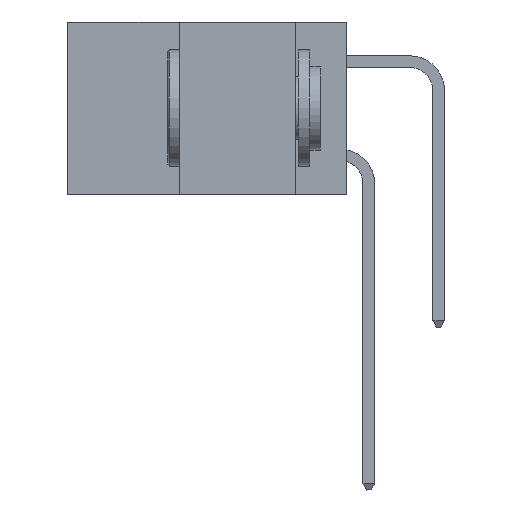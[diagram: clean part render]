
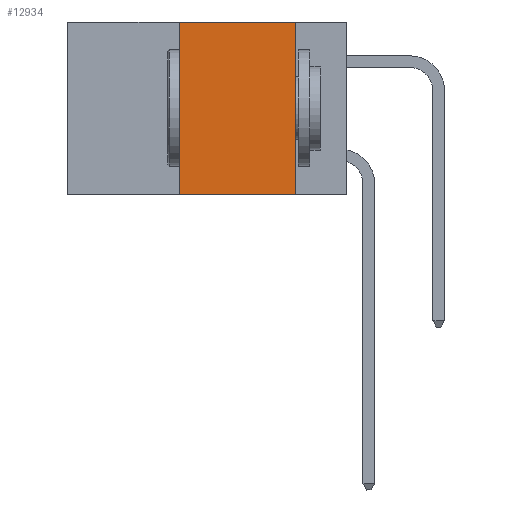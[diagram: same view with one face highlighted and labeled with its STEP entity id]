
A CAD part, left-side view. The second image highlights one B-rep face of the part: STEP entity #12934.
In plain terms, the highlighted planar face has unit normal (-1, 0, 0).
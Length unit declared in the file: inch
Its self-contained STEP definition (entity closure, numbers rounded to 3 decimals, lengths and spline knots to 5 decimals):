
#937 = LINE ( 'NONE', #5071, #10437 ) ;
#1653 = CARTESIAN_POINT ( 'NONE',  ( 0., 0.6, 0. ) ) ;
#1848 = CARTESIAN_POINT ( 'NONE',  ( 0., 0.36, 0. ) ) ;
#2266 = PLANE ( 'NONE',  #3835 ) ;
#2407 = ORIENTED_EDGE ( 'NONE', *, *, #3646, .F. ) ;
#2418 = CARTESIAN_POINT ( 'NONE',  ( 0., 0.11, 0. ) ) ;
#3545 = CARTESIAN_POINT ( 'NONE',  ( 0., 0.6, -0.37 ) ) ;
#3646 = EDGE_CURVE ( 'NONE', #12862, #16144, #12461, .T. ) ;
#3835 = AXIS2_PLACEMENT_3D ( 'NONE', #6542, #8156, #15404 ) ;
#4477 = EDGE_LOOP ( 'NONE', ( #12619, #5228, #2407, #12202 ) ) ;
#4644 = VECTOR ( 'NONE', #6473, 39.37008 ) ;
#5071 = CARTESIAN_POINT ( 'NONE',  ( 0., 0.11, 0. ) ) ;
#5228 = ORIENTED_EDGE ( 'NONE', *, *, #18281, .F. ) ;
#5990 = VECTOR ( 'NONE', #11857, 39.37008 ) ;
#6060 = VERTEX_POINT ( 'NONE', #8138 ) ;
#6473 = DIRECTION ( 'NONE',  ( 0., -1., 0. ) ) ;
#6542 = CARTESIAN_POINT ( 'NONE',  ( 0., 0.6, 0. ) ) ;
#7237 = VECTOR ( 'NONE', #7611, 39.37008 ) ;
#7611 = DIRECTION ( 'NONE',  ( 0., -1., 0. ) ) ;
#8138 = CARTESIAN_POINT ( 'NONE',  ( 0., 0.11, -0.37 ) ) ;
#8156 = DIRECTION ( 'NONE',  ( 1., 0., 0. ) ) ;
#9830 = VERTEX_POINT ( 'NONE', #2418 ) ;
#9888 = FACE_OUTER_BOUND ( 'NONE', #4477, .T. ) ;
#10437 = VECTOR ( 'NONE', #15437, 39.37008 ) ;
#11857 = DIRECTION ( 'NONE',  ( 0., 0., 1. ) ) ;
#12202 = ORIENTED_EDGE ( 'NONE', *, *, #15546, .T. ) ;
#12461 = LINE ( 'NONE', #13523, #5990 ) ;
#12619 = ORIENTED_EDGE ( 'NONE', *, *, #16235, .F. ) ;
#12862 = VERTEX_POINT ( 'NONE', #13082 ) ;
#12934 = ADVANCED_FACE ( 'NONE', ( #9888 ), #2266, .F. ) ;
#13082 = CARTESIAN_POINT ( 'NONE',  ( 0., 0.36, -0.37 ) ) ;
#13523 = CARTESIAN_POINT ( 'NONE',  ( 0., 0.36, 0. ) ) ;
#13930 = LINE ( 'NONE', #1653, #7237 ) ;
#15404 = DIRECTION ( 'NONE',  ( 0., 0., -1. ) ) ;
#15437 = DIRECTION ( 'NONE',  ( 0., 0., -1. ) ) ;
#15546 = EDGE_CURVE ( 'NONE', #12862, #6060, #16245, .T. ) ;
#16144 = VERTEX_POINT ( 'NONE', #1848 ) ;
#16235 = EDGE_CURVE ( 'NONE', #9830, #6060, #937, .T. ) ;
#16245 = LINE ( 'NONE', #3545, #4644 ) ;
#18281 = EDGE_CURVE ( 'NONE', #16144, #9830, #13930, .T. ) ;
